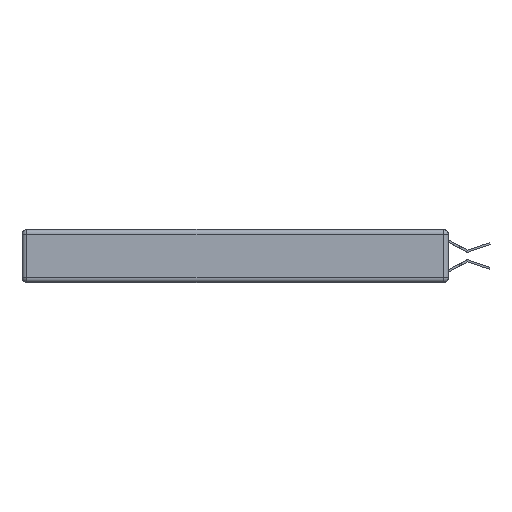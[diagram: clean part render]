
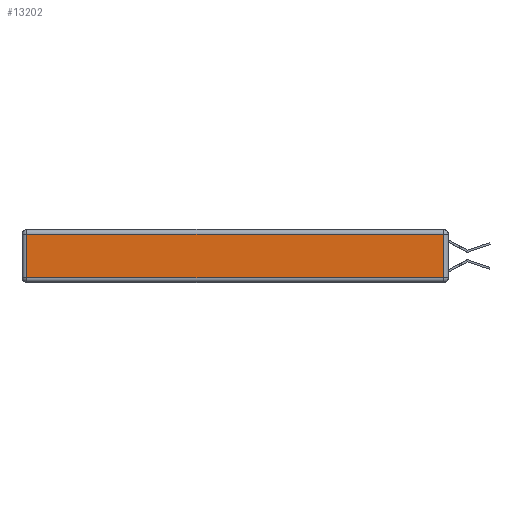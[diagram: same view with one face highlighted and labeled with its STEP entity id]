
A CAD part, left-side view. The second image highlights one B-rep face of the part: STEP entity #13202.
In plain terms, the highlighted planar face has unit normal (-1, 0, 0).
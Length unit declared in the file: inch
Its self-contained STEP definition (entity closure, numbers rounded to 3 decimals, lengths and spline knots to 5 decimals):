
#308 = ORIENTED_EDGE ( 'NONE', *, *, #10866, .T. ) ;
#538 = CARTESIAN_POINT ( 'NONE',  ( 0., 2.72, -0.313 ) ) ;
#741 = VERTEX_POINT ( 'NONE', #26421 ) ;
#1003 = CARTESIAN_POINT ( 'NONE',  ( 0., 0., -0.313 ) ) ;
#4792 = VECTOR ( 'NONE', #20374, 39.37008 ) ;
#5103 = DIRECTION ( 'NONE',  ( 0., 0., 1. ) ) ;
#5269 = DIRECTION ( 'NONE',  ( 0., 0., 1. ) ) ;
#5887 = ORIENTED_EDGE ( 'NONE', *, *, #7628, .T. ) ;
#6287 = CARTESIAN_POINT ( 'NONE',  ( 0., 2.75, -0.03 ) ) ;
#6500 = VERTEX_POINT ( 'NONE', #538 ) ;
#6934 = EDGE_LOOP ( 'NONE', ( #308, #22043, #5887, #25298 ) ) ;
#6967 = EDGE_CURVE ( 'NONE', #741, #26814, #7302, .T. ) ;
#7302 = LINE ( 'NONE', #13529, #17193 ) ;
#7628 = EDGE_CURVE ( 'NONE', #26814, #12929, #12251, .T. ) ;
#8103 = LINE ( 'NONE', #10414, #12799 ) ;
#10414 = CARTESIAN_POINT ( 'NONE',  ( 0., 2.72, -0.343 ) ) ;
#10866 = EDGE_CURVE ( 'NONE', #6500, #741, #12355, .T. ) ;
#12251 = LINE ( 'NONE', #6287, #18495 ) ;
#12355 = LINE ( 'NONE', #1003, #4792 ) ;
#12799 = VECTOR ( 'NONE', #20584, 39.37008 ) ;
#12929 = VERTEX_POINT ( 'NONE', #22498 ) ;
#13202 = ADVANCED_FACE ( 'NONE', ( #14751 ), #23022, .T. ) ;
#13529 = CARTESIAN_POINT ( 'NONE',  ( 0., 0.03, -0.343 ) ) ;
#14336 = DIRECTION ( 'NONE',  ( -1., 0., 0. ) ) ;
#14481 = CARTESIAN_POINT ( 'NONE',  ( 0., 0.03, -0.03 ) ) ;
#14751 = FACE_OUTER_BOUND ( 'NONE', #6934, .T. ) ;
#16130 = EDGE_CURVE ( 'NONE', #12929, #6500, #8103, .T. ) ;
#17193 = VECTOR ( 'NONE', #5269, 39.37008 ) ;
#18495 = VECTOR ( 'NONE', #20534, 39.37008 ) ;
#20374 = DIRECTION ( 'NONE',  ( 0., -1., 0. ) ) ;
#20534 = DIRECTION ( 'NONE',  ( 0., 1., 0. ) ) ;
#20584 = DIRECTION ( 'NONE',  ( 0., 0., -1. ) ) ;
#22043 = ORIENTED_EDGE ( 'NONE', *, *, #6967, .T. ) ;
#22498 = CARTESIAN_POINT ( 'NONE',  ( 0., 2.72, -0.03 ) ) ;
#23022 = PLANE ( 'NONE',  #25313 ) ;
#25298 = ORIENTED_EDGE ( 'NONE', *, *, #16130, .T. ) ;
#25313 = AXIS2_PLACEMENT_3D ( 'NONE', #25360, #14336, #5103 ) ;
#25360 = CARTESIAN_POINT ( 'NONE',  ( 0., 0., -0.343 ) ) ;
#26421 = CARTESIAN_POINT ( 'NONE',  ( 0., 0.03, -0.313 ) ) ;
#26814 = VERTEX_POINT ( 'NONE', #14481 ) ;
